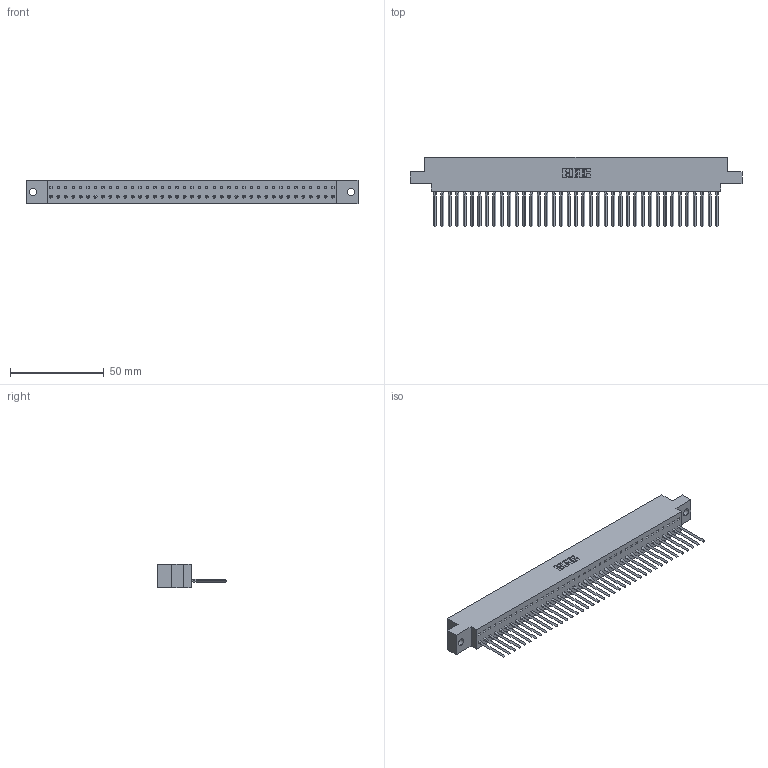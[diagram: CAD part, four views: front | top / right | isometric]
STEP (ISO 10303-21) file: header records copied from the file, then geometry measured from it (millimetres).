
FILE_DESCRIPTION (( 'STEP AP203' ), '1' );
FILE_NAME ('317-039-541-604.STEP', '2020-02-28T00:05:03', ( '' ), ( '' ), 'SwSTEP 2.0', 'SolidWorks 2016', '' );
FILE_SCHEMA (( 'CONFIG_CONTROL_DESIGN' ));
Length unit declared in the file: inch
Products named in the file (3): 317 Part_.156 Dia - TH; 317-039-541-604; 317-290-002_541
Assembly tree (40 placements, depth 2):
  317-039-541-604
    317 Part_.156 Dia - TH
    317-290-002_541  x39
Bounding box: 177.24 x 37.34 x 12.7 mm (x, y, z)
Volume: 28562.5 mm3; surface area: 40078.6 mm2
Topology: 40 solids, 40 shells, 6030 faces, 17201 edges, 11180 vertices
Faces by surface type: plane 4894, cylinder 980, bspline 156
Entity records: 57096 total; most frequent: CARTESIAN_POINT 10790, ORIENTED_EDGE 10082, DIRECTION 8279, EDGE_CURVE 5041, LINE 4677, VECTOR 4677, VERTEX_POINT 3352, AXIS2_PLACEMENT_3D 1801
